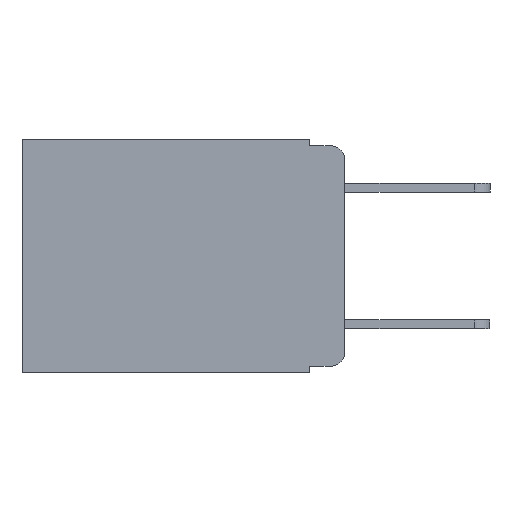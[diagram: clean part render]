
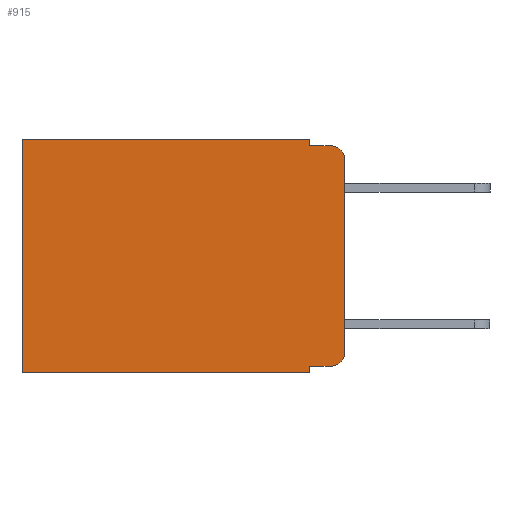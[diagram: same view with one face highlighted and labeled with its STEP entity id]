
A CAD part, left-side view. The second image highlights one B-rep face of the part: STEP entity #915.
In plain terms, the highlighted planar face has unit normal (-1, 0, 0).
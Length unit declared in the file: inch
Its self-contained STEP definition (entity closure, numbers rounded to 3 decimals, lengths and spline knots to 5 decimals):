
#146 = FACE_OUTER_BOUND ( 'NONE', #23984, .T. ) ;
#168 = LINE ( 'NONE', #18640, #19470 ) ;
#263 = LINE ( 'NONE', #7311, #15893 ) ;
#298 = EDGE_CURVE ( 'NONE', #7194, #10943, #13232, .T. ) ;
#454 = PLANE ( 'NONE',  #18701 ) ;
#519 = CARTESIAN_POINT ( 'NONE',  ( 0.298, 0., -0.343 ) ) ;
#915 = ADVANCED_FACE ( 'NONE', ( #146 ), #454, .F. ) ;
#973 = VERTEX_POINT ( 'NONE', #980 ) ;
#980 = CARTESIAN_POINT ( 'NONE',  ( 0.298, 0., -0.03 ) ) ;
#1671 = VERTEX_POINT ( 'NONE', #16214 ) ;
#1779 = CARTESIAN_POINT ( 'NONE',  ( 0.298, 0., 0. ) ) ;
#2367 = CARTESIAN_POINT ( 'NONE',  ( 0.298, 0.02, -0.01 ) ) ;
#2516 = DIRECTION ( 'NONE',  ( 0., 1., 0. ) ) ;
#2673 = VECTOR ( 'NONE', #13524, 39.37008 ) ;
#2864 = DIRECTION ( 'NONE',  ( 0., 1., 0. ) ) ;
#3219 = EDGE_CURVE ( 'NONE', #973, #15645, #5862, .T. ) ;
#3398 = DIRECTION ( 'NONE',  ( 0., 0., -1. ) ) ;
#4170 = CARTESIAN_POINT ( 'NONE',  ( 0.298, 0.02, -0.03 ) ) ;
#4197 = ORIENTED_EDGE ( 'NONE', *, *, #8301, .T. ) ;
#4380 = DIRECTION ( 'NONE',  ( -1., 0., 0. ) ) ;
#4730 = DIRECTION ( 'NONE',  ( 0., 0., -1. ) ) ;
#4820 = CARTESIAN_POINT ( 'NONE',  ( 0.298, 0.051, 0. ) ) ;
#4864 = ORIENTED_EDGE ( 'NONE', *, *, #3219, .T. ) ;
#4998 = DIRECTION ( 'NONE',  ( 1., 0., 0. ) ) ;
#5006 = VECTOR ( 'NONE', #7664, 39.37008 ) ;
#5296 = VERTEX_POINT ( 'NONE', #11926 ) ;
#5603 = LINE ( 'NONE', #22302, #5006 ) ;
#5782 = EDGE_CURVE ( 'NONE', #5296, #15645, #263, .T. ) ;
#5862 = CIRCLE ( 'NONE', #22809, 0.02 ) ;
#6277 = ORIENTED_EDGE ( 'NONE', *, *, #21774, .T. ) ;
#6373 = LINE ( 'NONE', #4820, #19886 ) ;
#6865 = ORIENTED_EDGE ( 'NONE', *, *, #298, .T. ) ;
#7025 = EDGE_CURVE ( 'NONE', #7194, #5296, #22899, .T. ) ;
#7194 = VERTEX_POINT ( 'NONE', #18392 ) ;
#7311 = CARTESIAN_POINT ( 'NONE',  ( 0.298, 0.051, -0.01 ) ) ;
#7522 = DIRECTION ( 'NONE',  ( 0., -1., 0. ) ) ;
#7664 = DIRECTION ( 'NONE',  ( 0., 0., -1. ) ) ;
#7972 = CARTESIAN_POINT ( 'NONE',  ( 0.298, 0., -0.313 ) ) ;
#8301 = EDGE_CURVE ( 'NONE', #10943, #8415, #168, .T. ) ;
#8328 = ORIENTED_EDGE ( 'NONE', *, *, #5782, .F. ) ;
#8415 = VERTEX_POINT ( 'NONE', #22929 ) ;
#9112 = DIRECTION ( 'NONE',  ( -1., 0., 0. ) ) ;
#9315 = LINE ( 'NONE', #519, #18503 ) ;
#10737 = EDGE_CURVE ( 'NONE', #21308, #1671, #6373, .T. ) ;
#10753 = CARTESIAN_POINT ( 'NONE',  ( 0.298, 0.051, -0.333 ) ) ;
#10845 = CIRCLE ( 'NONE', #17476, 0.02 ) ;
#10943 = VERTEX_POINT ( 'NONE', #23635 ) ;
#11812 = ORIENTED_EDGE ( 'NONE', *, *, #18587, .F. ) ;
#11926 = CARTESIAN_POINT ( 'NONE',  ( 0.298, 0.051, -0.01 ) ) ;
#11998 = EDGE_CURVE ( 'NONE', #21308, #12171, #17847, .T. ) ;
#12171 = VERTEX_POINT ( 'NONE', #17909 ) ;
#12965 = ORIENTED_EDGE ( 'NONE', *, *, #23380, .F. ) ;
#13232 = LINE ( 'NONE', #1779, #17500 ) ;
#13524 = DIRECTION ( 'NONE',  ( 0., 0., -1. ) ) ;
#13581 = CARTESIAN_POINT ( 'NONE',  ( 0.298, 0.051, 0. ) ) ;
#15406 = CARTESIAN_POINT ( 'NONE',  ( 0.298, 0., 0. ) ) ;
#15645 = VERTEX_POINT ( 'NONE', #2367 ) ;
#15734 = ORIENTED_EDGE ( 'NONE', *, *, #11998, .T. ) ;
#15893 = VECTOR ( 'NONE', #7522, 39.37008 ) ;
#15974 = DIRECTION ( 'NONE',  ( 0., 0., -1. ) ) ;
#16214 = CARTESIAN_POINT ( 'NONE',  ( 0.298, 0.051, -0.343 ) ) ;
#17285 = VECTOR ( 'NONE', #22904, 39.37008 ) ;
#17476 = AXIS2_PLACEMENT_3D ( 'NONE', #20083, #9112, #21906 ) ;
#17500 = VECTOR ( 'NONE', #2864, 39.37008 ) ;
#17847 = LINE ( 'NONE', #21073, #17285 ) ;
#17909 = CARTESIAN_POINT ( 'NONE',  ( 0.298, 0.02, -0.333 ) ) ;
#18392 = CARTESIAN_POINT ( 'NONE',  ( 0.298, 0.051, 0. ) ) ;
#18503 = VECTOR ( 'NONE', #2516, 39.37008 ) ;
#18587 = EDGE_CURVE ( 'NONE', #973, #20971, #5603, .T. ) ;
#18640 = CARTESIAN_POINT ( 'NONE',  ( 0.298, 0.473, 0. ) ) ;
#18701 = AXIS2_PLACEMENT_3D ( 'NONE', #15406, #4998, #15974 ) ;
#19470 = VECTOR ( 'NONE', #21965, 39.37008 ) ;
#19886 = VECTOR ( 'NONE', #4730, 39.37008 ) ;
#20059 = ORIENTED_EDGE ( 'NONE', *, *, #10737, .F. ) ;
#20083 = CARTESIAN_POINT ( 'NONE',  ( 0.298, 0.02, -0.313 ) ) ;
#20871 = ORIENTED_EDGE ( 'NONE', *, *, #7025, .F. ) ;
#20971 = VERTEX_POINT ( 'NONE', #7972 ) ;
#21073 = CARTESIAN_POINT ( 'NONE',  ( 0.298, 0.051, -0.333 ) ) ;
#21308 = VERTEX_POINT ( 'NONE', #10753 ) ;
#21774 = EDGE_CURVE ( 'NONE', #12171, #20971, #10845, .T. ) ;
#21906 = DIRECTION ( 'NONE',  ( 0., 0., -1. ) ) ;
#21965 = DIRECTION ( 'NONE',  ( 0., 0., -1. ) ) ;
#22302 = CARTESIAN_POINT ( 'NONE',  ( 0.298, 0., 0. ) ) ;
#22809 = AXIS2_PLACEMENT_3D ( 'NONE', #4170, #4380, #3398 ) ;
#22899 = LINE ( 'NONE', #13581, #2673 ) ;
#22904 = DIRECTION ( 'NONE',  ( 0., -1., 0. ) ) ;
#22929 = CARTESIAN_POINT ( 'NONE',  ( 0.298, 0.473, -0.343 ) ) ;
#23380 = EDGE_CURVE ( 'NONE', #1671, #8415, #9315, .T. ) ;
#23635 = CARTESIAN_POINT ( 'NONE',  ( 0.298, 0.473, 0. ) ) ;
#23984 = EDGE_LOOP ( 'NONE', ( #11812, #4864, #8328, #20871, #6865, #4197, #12965, #20059, #15734, #6277 ) ) ;
